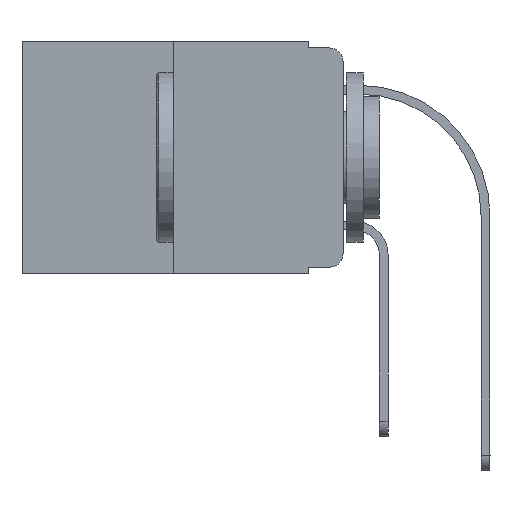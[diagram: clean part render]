
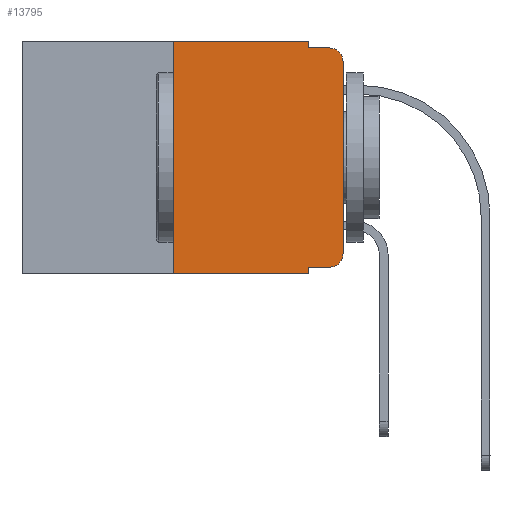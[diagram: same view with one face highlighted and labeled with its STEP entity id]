
A CAD part, left-side view. The second image highlights one B-rep face of the part: STEP entity #13795.
In plain terms, the highlighted planar face has unit normal (-1, 0, 0).
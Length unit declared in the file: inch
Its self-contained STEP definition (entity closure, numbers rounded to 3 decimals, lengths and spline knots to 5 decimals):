
#79 = VERTEX_POINT ( 'NONE', #1661 ) ;
#446 = EDGE_CURVE ( 'NONE', #11268, #79, #4912, .T. ) ;
#538 = DIRECTION ( 'NONE',  ( 0., 0., -1. ) ) ;
#540 = DIRECTION ( 'NONE',  ( 0., 0., -1. ) ) ;
#664 = VERTEX_POINT ( 'NONE', #11012 ) ;
#892 = CARTESIAN_POINT ( 'NONE',  ( 0., 0.25, -0.343 ) ) ;
#1018 = DIRECTION ( 'NONE',  ( 1., 0., 0. ) ) ;
#1073 = CIRCLE ( 'NONE', #10022, 0.02 ) ;
#1287 = AXIS2_PLACEMENT_3D ( 'NONE', #11128, #1018, #14551 ) ;
#1369 = VECTOR ( 'NONE', #10675, 39.37008 ) ;
#1534 = DIRECTION ( 'NONE',  ( 0., 0., 1. ) ) ;
#1635 = VECTOR ( 'NONE', #6567, 39.37008 ) ;
#1661 = CARTESIAN_POINT ( 'NONE',  ( 0., 0.051, -0.343 ) ) ;
#2078 = DIRECTION ( 'NONE',  ( 0., -1., 0. ) ) ;
#2237 = ORIENTED_EDGE ( 'NONE', *, *, #446, .F. ) ;
#2262 = CARTESIAN_POINT ( 'NONE',  ( 0., 0.02, -0.01 ) ) ;
#2811 = ORIENTED_EDGE ( 'NONE', *, *, #3939, .F. ) ;
#2908 = VECTOR ( 'NONE', #4361, 39.37008 ) ;
#3212 = LINE ( 'NONE', #10084, #1635 ) ;
#3221 = CARTESIAN_POINT ( 'NONE',  ( 0., 0., -0.03 ) ) ;
#3592 = CARTESIAN_POINT ( 'NONE',  ( 0., 0.473, -0.343 ) ) ;
#3796 = CARTESIAN_POINT ( 'NONE',  ( 0., 0.051, 0. ) ) ;
#3939 = EDGE_CURVE ( 'NONE', #9288, #12491, #10443, .T. ) ;
#3965 = VERTEX_POINT ( 'NONE', #3221 ) ;
#4299 = VERTEX_POINT ( 'NONE', #13773 ) ;
#4361 = DIRECTION ( 'NONE',  ( 0., -1., 0. ) ) ;
#4409 = ORIENTED_EDGE ( 'NONE', *, *, #12020, .F. ) ;
#4550 = ORIENTED_EDGE ( 'NONE', *, *, #11400, .T. ) ;
#4566 = CARTESIAN_POINT ( 'NONE',  ( 0., 0.051, -0.333 ) ) ;
#4912 = LINE ( 'NONE', #3796, #11557 ) ;
#5159 = VERTEX_POINT ( 'NONE', #5837 ) ;
#5458 = ORIENTED_EDGE ( 'NONE', *, *, #11752, .T. ) ;
#5525 = VECTOR ( 'NONE', #1534, 39.37008 ) ;
#5749 = LINE ( 'NONE', #11126, #2908 ) ;
#5798 = VECTOR ( 'NONE', #9557, 39.37008 ) ;
#5837 = CARTESIAN_POINT ( 'NONE',  ( 0., 0.25, 0. ) ) ;
#5900 = EDGE_LOOP ( 'NONE', ( #4550, #5458, #2811, #11234, #4409, #7518, #9979, #2237, #10666, #8303 ) ) ;
#5901 = CARTESIAN_POINT ( 'NONE',  ( 0., 0.25, 0. ) ) ;
#6094 = CARTESIAN_POINT ( 'NONE',  ( 0., 0.02, -0.03 ) ) ;
#6187 = CARTESIAN_POINT ( 'NONE',  ( 0., 0., 0. ) ) ;
#6189 = CARTESIAN_POINT ( 'NONE',  ( 0., 0.051, -0.01 ) ) ;
#6567 = DIRECTION ( 'NONE',  ( 0., 0., -1. ) ) ;
#6765 = EDGE_CURVE ( 'NONE', #4299, #9288, #3212, .T. ) ;
#7518 = ORIENTED_EDGE ( 'NONE', *, *, #8377, .F. ) ;
#7675 = CARTESIAN_POINT ( 'NONE',  ( 0., 0.051, -0.01 ) ) ;
#7962 = DIRECTION ( 'NONE',  ( 0., -1., 0. ) ) ;
#8154 = EDGE_CURVE ( 'NONE', #11268, #664, #5749, .T. ) ;
#8303 = ORIENTED_EDGE ( 'NONE', *, *, #11870, .T. ) ;
#8377 = EDGE_CURVE ( 'NONE', #8929, #5159, #10305, .T. ) ;
#8405 = VECTOR ( 'NONE', #2078, 39.37008 ) ;
#8840 = PLANE ( 'NONE',  #1287 ) ;
#8929 = VERTEX_POINT ( 'NONE', #892 ) ;
#9288 = VERTEX_POINT ( 'NONE', #7675 ) ;
#9557 = DIRECTION ( 'NONE',  ( 0., 0., 1. ) ) ;
#9979 = ORIENTED_EDGE ( 'NONE', *, *, #11179, .T. ) ;
#10009 = FACE_OUTER_BOUND ( 'NONE', #5900, .T. ) ;
#10022 = AXIS2_PLACEMENT_3D ( 'NONE', #6094, #10572, #10263 ) ;
#10084 = CARTESIAN_POINT ( 'NONE',  ( 0., 0.051, 0. ) ) ;
#10224 = CARTESIAN_POINT ( 'NONE',  ( 0., 0.473, 0. ) ) ;
#10263 = DIRECTION ( 'NONE',  ( 0., 0., -1. ) ) ;
#10305 = LINE ( 'NONE', #5901, #5525 ) ;
#10443 = LINE ( 'NONE', #6189, #1369 ) ;
#10572 = DIRECTION ( 'NONE',  ( -1., 0., 0. ) ) ;
#10666 = ORIENTED_EDGE ( 'NONE', *, *, #8154, .T. ) ;
#10675 = DIRECTION ( 'NONE',  ( 0., -1., 0. ) ) ;
#10964 = VECTOR ( 'NONE', #7962, 39.37008 ) ;
#11012 = CARTESIAN_POINT ( 'NONE',  ( 0., 0.02, -0.333 ) ) ;
#11126 = CARTESIAN_POINT ( 'NONE',  ( 0., 0.051, -0.333 ) ) ;
#11128 = CARTESIAN_POINT ( 'NONE',  ( 0., 0.473, 0. ) ) ;
#11179 = EDGE_CURVE ( 'NONE', #8929, #79, #11271, .T. ) ;
#11234 = ORIENTED_EDGE ( 'NONE', *, *, #6765, .F. ) ;
#11268 = VERTEX_POINT ( 'NONE', #4566 ) ;
#11271 = LINE ( 'NONE', #3592, #10964 ) ;
#11400 = EDGE_CURVE ( 'NONE', #11552, #3965, #13787, .T. ) ;
#11552 = VERTEX_POINT ( 'NONE', #12151 ) ;
#11557 = VECTOR ( 'NONE', #540, 39.37008 ) ;
#11752 = EDGE_CURVE ( 'NONE', #3965, #12491, #1073, .T. ) ;
#11870 = EDGE_CURVE ( 'NONE', #664, #11552, #12177, .T. ) ;
#12020 = EDGE_CURVE ( 'NONE', #5159, #4299, #13372, .T. ) ;
#12059 = CARTESIAN_POINT ( 'NONE',  ( 0., 0.02, -0.313 ) ) ;
#12151 = CARTESIAN_POINT ( 'NONE',  ( 0., 0., -0.313 ) ) ;
#12177 = CIRCLE ( 'NONE', #13825, 0.02 ) ;
#12491 = VERTEX_POINT ( 'NONE', #2262 ) ;
#13085 = DIRECTION ( 'NONE',  ( -1., 0., 0. ) ) ;
#13372 = LINE ( 'NONE', #10224, #8405 ) ;
#13773 = CARTESIAN_POINT ( 'NONE',  ( 0., 0.051, 0. ) ) ;
#13787 = LINE ( 'NONE', #6187, #5798 ) ;
#13795 = ADVANCED_FACE ( 'NONE', ( #10009 ), #8840, .F. ) ;
#13825 = AXIS2_PLACEMENT_3D ( 'NONE', #12059, #13085, #538 ) ;
#14551 = DIRECTION ( 'NONE',  ( 0., 0., -1. ) ) ;
